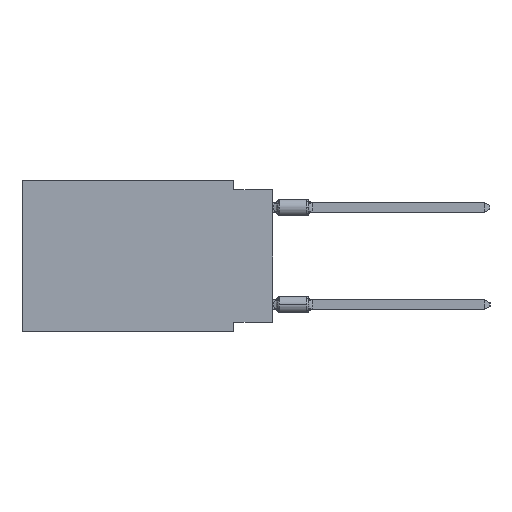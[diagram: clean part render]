
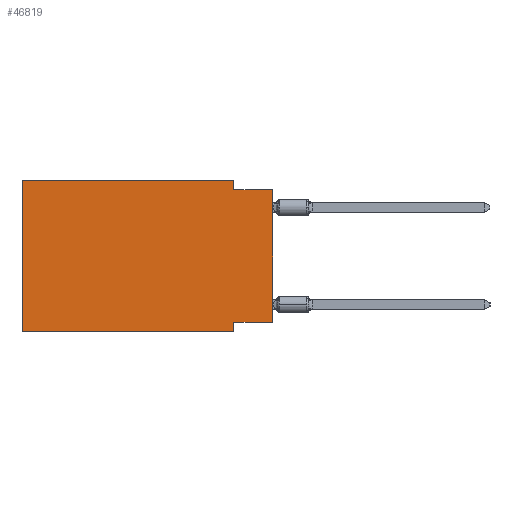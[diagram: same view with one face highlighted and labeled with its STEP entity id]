
A CAD part, left-side view. The second image highlights one B-rep face of the part: STEP entity #46819.
In plain terms, the highlighted planar face has unit normal (-1, 0, 0).
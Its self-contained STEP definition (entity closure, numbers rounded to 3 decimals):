
#220 = VERTEX_POINT ( 'NONE', #19990 ) ;
#624 = CARTESIAN_POINT ( 'NONE',  ( 0., 16.383, 0. ) ) ;
#719 = VERTEX_POINT ( 'NONE', #33354 ) ;
#1392 = VERTEX_POINT ( 'NONE', #31567 ) ;
#1431 = LINE ( 'NONE', #40411, #28229 ) ;
#1936 = VECTOR ( 'NONE', #17296, 1000. ) ;
#3502 = CARTESIAN_POINT ( 'NONE',  ( 0., 2.54, 0. ) ) ;
#5581 = VECTOR ( 'NONE', #45808, 1000. ) ;
#7085 = EDGE_LOOP ( 'NONE', ( #38241, #25759, #35359, #24333, #24269, #39897, #17827, #54810 ) ) ;
#9015 = LINE ( 'NONE', #35174, #52237 ) ;
#9262 = DIRECTION ( 'NONE',  ( 0., 0., 1. ) ) ;
#10150 = VECTOR ( 'NONE', #44166, 1000. ) ;
#11191 = CARTESIAN_POINT ( 'NONE',  ( 0., 2.54, -9.271 ) ) ;
#12433 = DIRECTION ( 'NONE',  ( 0., 0., -1. ) ) ;
#13393 = CARTESIAN_POINT ( 'NONE',  ( 0., 0., -9.271 ) ) ;
#13526 = VERTEX_POINT ( 'NONE', #43824 ) ;
#14993 = EDGE_CURVE ( 'NONE', #13526, #220, #25121, .T. ) ;
#15670 = LINE ( 'NONE', #50436, #28235 ) ;
#16031 = LINE ( 'NONE', #41367, #5581 ) ;
#16344 = DIRECTION ( 'NONE',  ( 1., 0., 0. ) ) ;
#16795 = LINE ( 'NONE', #624, #24577 ) ;
#17296 = DIRECTION ( 'NONE',  ( 0., -1., 0. ) ) ;
#17827 = ORIENTED_EDGE ( 'NONE', *, *, #52366, .F. ) ;
#19990 = CARTESIAN_POINT ( 'NONE',  ( 0., 2.54, -9.906 ) ) ;
#20130 = DIRECTION ( 'NONE',  ( 0., -1., 0. ) ) ;
#20388 = EDGE_CURVE ( 'NONE', #36535, #54811, #31369, .T. ) ;
#24269 = ORIENTED_EDGE ( 'NONE', *, *, #30930, .F. ) ;
#24333 = ORIENTED_EDGE ( 'NONE', *, *, #20388, .F. ) ;
#24577 = VECTOR ( 'NONE', #9262, 1000. ) ;
#25121 = LINE ( 'NONE', #45474, #50822 ) ;
#25759 = ORIENTED_EDGE ( 'NONE', *, *, #47735, .F. ) ;
#27446 = CARTESIAN_POINT ( 'NONE',  ( 0., 16.383, 0. ) ) ;
#28229 = VECTOR ( 'NONE', #52639, 1000. ) ;
#28235 = VECTOR ( 'NONE', #41015, 1000. ) ;
#30930 = EDGE_CURVE ( 'NONE', #13526, #36535, #16795, .T. ) ;
#31369 = LINE ( 'NONE', #27446, #10150 ) ;
#31567 = CARTESIAN_POINT ( 'NONE',  ( 0., 2.54, -0.635 ) ) ;
#33045 = PLANE ( 'NONE',  #36549 ) ;
#33354 = CARTESIAN_POINT ( 'NONE',  ( 0., 0., -0.635 ) ) ;
#35174 = CARTESIAN_POINT ( 'NONE',  ( 0., 2.54, 0. ) ) ;
#35359 = ORIENTED_EDGE ( 'NONE', *, *, #52181, .F. ) ;
#36535 = VERTEX_POINT ( 'NONE', #52670 ) ;
#36549 = AXIS2_PLACEMENT_3D ( 'NONE', #46374, #16344, #12433 ) ;
#37904 = CARTESIAN_POINT ( 'NONE',  ( 0., 0., -0.635 ) ) ;
#38241 = ORIENTED_EDGE ( 'NONE', *, *, #42466, .T. ) ;
#38729 = LINE ( 'NONE', #37904, #1936 ) ;
#39671 = VERTEX_POINT ( 'NONE', #13393 ) ;
#39897 = ORIENTED_EDGE ( 'NONE', *, *, #14993, .T. ) ;
#40411 = CARTESIAN_POINT ( 'NONE',  ( 0., 0., -9.271 ) ) ;
#41015 = DIRECTION ( 'NONE',  ( 0., 0., -1. ) ) ;
#41367 = CARTESIAN_POINT ( 'NONE',  ( 0., 0., 0. ) ) ;
#42466 = EDGE_CURVE ( 'NONE', #39671, #719, #16031, .T. ) ;
#43824 = CARTESIAN_POINT ( 'NONE',  ( 0., 16.383, -9.906 ) ) ;
#44166 = DIRECTION ( 'NONE',  ( 0., -1., 0. ) ) ;
#45474 = CARTESIAN_POINT ( 'NONE',  ( 0., 16.383, -9.906 ) ) ;
#45808 = DIRECTION ( 'NONE',  ( 0., 0., 1. ) ) ;
#46374 = CARTESIAN_POINT ( 'NONE',  ( 0., 16.383, 0. ) ) ;
#46819 = ADVANCED_FACE ( 'NONE', ( #50550 ), #33045, .F. ) ;
#47735 = EDGE_CURVE ( 'NONE', #1392, #719, #38729, .T. ) ;
#48362 = VERTEX_POINT ( 'NONE', #11191 ) ;
#50436 = CARTESIAN_POINT ( 'NONE',  ( 0., 2.54, -9.906 ) ) ;
#50550 = FACE_OUTER_BOUND ( 'NONE', #7085, .T. ) ;
#50822 = VECTOR ( 'NONE', #20130, 1000. ) ;
#51605 = DIRECTION ( 'NONE',  ( 0., 0., -1. ) ) ;
#52181 = EDGE_CURVE ( 'NONE', #54811, #1392, #9015, .T. ) ;
#52237 = VECTOR ( 'NONE', #51605, 1000. ) ;
#52366 = EDGE_CURVE ( 'NONE', #48362, #220, #15670, .T. ) ;
#52639 = DIRECTION ( 'NONE',  ( 0., 1., 0. ) ) ;
#52670 = CARTESIAN_POINT ( 'NONE',  ( 0., 16.383, 0. ) ) ;
#53843 = EDGE_CURVE ( 'NONE', #39671, #48362, #1431, .T. ) ;
#54810 = ORIENTED_EDGE ( 'NONE', *, *, #53843, .F. ) ;
#54811 = VERTEX_POINT ( 'NONE', #3502 ) ;
